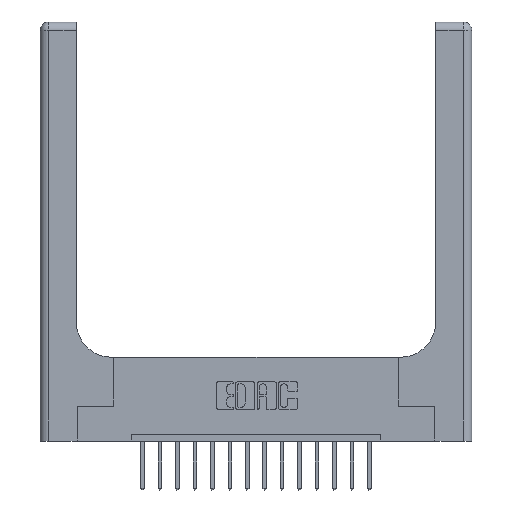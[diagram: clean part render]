
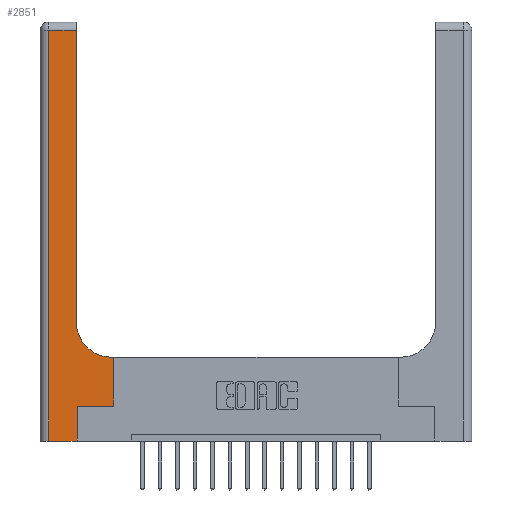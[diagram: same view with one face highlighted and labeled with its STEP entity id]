
A CAD part, top view. The second image highlights one B-rep face of the part: STEP entity #2851.
In plain terms, the highlighted planar face has unit normal (0, 0, 1).
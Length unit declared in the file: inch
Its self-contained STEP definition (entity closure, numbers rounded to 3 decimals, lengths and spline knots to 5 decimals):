
#788 = DIRECTION ( 'NONE',  ( -1., 0., 0. ) ) ;
#873 = LINE ( 'NONE', #13494, #7712 ) ;
#898 = CARTESIAN_POINT ( 'NONE',  ( 0., 2.94, 0.37 ) ) ;
#912 = ORIENTED_EDGE ( 'NONE', *, *, #6438, .T. ) ;
#1521 = DIRECTION ( 'NONE',  ( 0., -1., 0. ) ) ;
#2175 = LINE ( 'NONE', #898, #4429 ) ;
#2368 = LINE ( 'NONE', #2463, #6725 ) ;
#2387 = CARTESIAN_POINT ( 'NONE',  ( 0.265, 0., 0.37 ) ) ;
#2463 = CARTESIAN_POINT ( 'NONE',  ( 0.528, 0.25, 0.37 ) ) ;
#2484 = ORIENTED_EDGE ( 'NONE', *, *, #15612, .T. ) ;
#2545 = DIRECTION ( 'NONE',  ( 0., 1., 0. ) ) ;
#2692 = CIRCLE ( 'NONE', #17606, 0.25 ) ;
#2793 = LINE ( 'NONE', #18005, #10481 ) ;
#2851 = ADVANCED_FACE ( 'NONE', ( #13618 ), #10609, .F. ) ;
#2857 = DIRECTION ( 'NONE',  ( 0., 0., -1. ) ) ;
#3170 = VERTEX_POINT ( 'NONE', #9918 ) ;
#4388 = VECTOR ( 'NONE', #4721, 39.37008 ) ;
#4429 = VECTOR ( 'NONE', #13336, 39.37008 ) ;
#4557 = CARTESIAN_POINT ( 'NONE',  ( 0.51, 0.6, 0.37 ) ) ;
#4609 = VECTOR ( 'NONE', #788, 39.37008 ) ;
#4721 = DIRECTION ( 'NONE',  ( 0., 1., 0. ) ) ;
#4884 = DIRECTION ( 'NONE',  ( 1., 0., 0. ) ) ;
#5030 = EDGE_CURVE ( 'NONE', #15999, #11970, #873, .T. ) ;
#5568 = VERTEX_POINT ( 'NONE', #9966 ) ;
#5616 = VERTEX_POINT ( 'NONE', #4557 ) ;
#5755 = EDGE_LOOP ( 'NONE', ( #8195, #2484, #6922, #8954, #11603, #13418, #13916, #10835, #912 ) ) ;
#5923 = EDGE_CURVE ( 'NONE', #3170, #15999, #2793, .T. ) ;
#6438 = EDGE_CURVE ( 'NONE', #5616, #5568, #2692, .T. ) ;
#6725 = VECTOR ( 'NONE', #2545, 39.37008 ) ;
#6922 = ORIENTED_EDGE ( 'NONE', *, *, #5923, .T. ) ;
#7712 = VECTOR ( 'NONE', #4884, 39.37008 ) ;
#7751 = EDGE_CURVE ( 'NONE', #9705, #15622, #2368, .T. ) ;
#8037 = DIRECTION ( 'NONE',  ( -1., 0., 0. ) ) ;
#8108 = CARTESIAN_POINT ( 'NONE',  ( 0.528, 0.6, 0.37 ) ) ;
#8195 = ORIENTED_EDGE ( 'NONE', *, *, #12472, .T. ) ;
#8954 = ORIENTED_EDGE ( 'NONE', *, *, #5030, .T. ) ;
#9409 = CARTESIAN_POINT ( 'NONE',  ( 0.265, 0.25, 0.37 ) ) ;
#9705 = VERTEX_POINT ( 'NONE', #12033 ) ;
#9785 = EDGE_CURVE ( 'NONE', #15622, #5616, #10574, .T. ) ;
#9918 = CARTESIAN_POINT ( 'NONE',  ( 0.06, 2.94, 0.37 ) ) ;
#9966 = CARTESIAN_POINT ( 'NONE',  ( 0.26, 0.85, 0.37 ) ) ;
#10315 = DIRECTION ( 'NONE',  ( 1., 0., 0. ) ) ;
#10481 = VECTOR ( 'NONE', #1521, 39.37008 ) ;
#10574 = LINE ( 'NONE', #13496, #4609 ) ;
#10609 = PLANE ( 'NONE',  #16149 ) ;
#10620 = VECTOR ( 'NONE', #10315, 39.37008 ) ;
#10835 = ORIENTED_EDGE ( 'NONE', *, *, #9785, .T. ) ;
#11012 = CARTESIAN_POINT ( 'NONE',  ( 0.26, 2.94, 0.37 ) ) ;
#11513 = CARTESIAN_POINT ( 'NONE',  ( 0.26, 3., 0.37 ) ) ;
#11603 = ORIENTED_EDGE ( 'NONE', *, *, #16771, .T. ) ;
#11795 = LINE ( 'NONE', #17383, #17618 ) ;
#11970 = VERTEX_POINT ( 'NONE', #2387 ) ;
#12033 = CARTESIAN_POINT ( 'NONE',  ( 0.528, 0.25, 0.37 ) ) ;
#12472 = EDGE_CURVE ( 'NONE', #5568, #14488, #17278, .T. ) ;
#13336 = DIRECTION ( 'NONE',  ( -1., 0., 0. ) ) ;
#13418 = ORIENTED_EDGE ( 'NONE', *, *, #17211, .T. ) ;
#13494 = CARTESIAN_POINT ( 'NONE',  ( 0., 0., 0.37 ) ) ;
#13496 = CARTESIAN_POINT ( 'NONE',  ( 0.26, 0.6, 0.37 ) ) ;
#13618 = FACE_OUTER_BOUND ( 'NONE', #5755, .T. ) ;
#13916 = ORIENTED_EDGE ( 'NONE', *, *, #7751, .T. ) ;
#14488 = VERTEX_POINT ( 'NONE', #11012 ) ;
#15612 = EDGE_CURVE ( 'NONE', #14488, #3170, #2175, .T. ) ;
#15622 = VERTEX_POINT ( 'NONE', #8108 ) ;
#15772 = DIRECTION ( 'NONE',  ( 1., 0., 0. ) ) ;
#15896 = CARTESIAN_POINT ( 'NONE',  ( 0.06, 0., 0.37 ) ) ;
#15999 = VERTEX_POINT ( 'NONE', #15896 ) ;
#16149 = AXIS2_PLACEMENT_3D ( 'NONE', #17830, #16372, #8037 ) ;
#16196 = DIRECTION ( 'NONE',  ( 0., 1., 0. ) ) ;
#16372 = DIRECTION ( 'NONE',  ( 0., 0., -1. ) ) ;
#16771 = EDGE_CURVE ( 'NONE', #11970, #16901, #11795, .T. ) ;
#16901 = VERTEX_POINT ( 'NONE', #9409 ) ;
#17063 = CARTESIAN_POINT ( 'NONE',  ( 0.51, 0.85, 0.37 ) ) ;
#17093 = CARTESIAN_POINT ( 'NONE',  ( 0.265, 0.25, 0.37 ) ) ;
#17211 = EDGE_CURVE ( 'NONE', #16901, #9705, #17268, .T. ) ;
#17268 = LINE ( 'NONE', #17093, #10620 ) ;
#17278 = LINE ( 'NONE', #11513, #4388 ) ;
#17383 = CARTESIAN_POINT ( 'NONE',  ( 0.265, 0., 0.37 ) ) ;
#17606 = AXIS2_PLACEMENT_3D ( 'NONE', #17063, #2857, #15772 ) ;
#17618 = VECTOR ( 'NONE', #16196, 39.37008 ) ;
#17830 = CARTESIAN_POINT ( 'NONE',  ( 0., 3., 0.37 ) ) ;
#18005 = CARTESIAN_POINT ( 'NONE',  ( 0.06, 3., 0.37 ) ) ;
